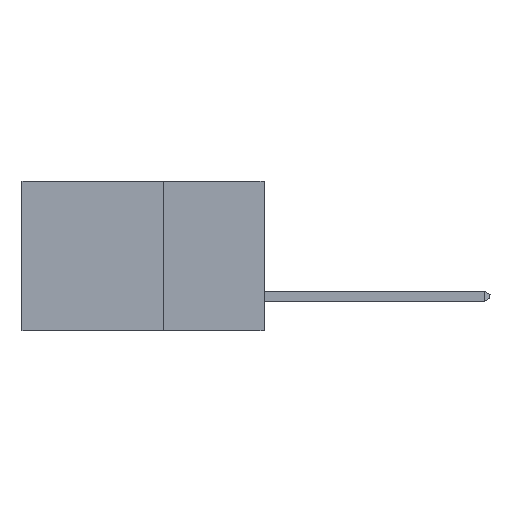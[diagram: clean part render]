
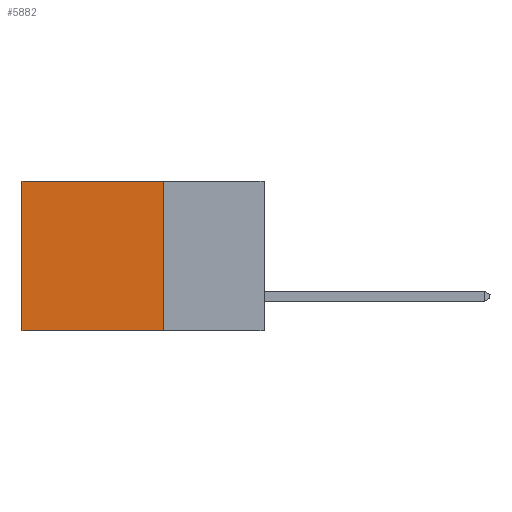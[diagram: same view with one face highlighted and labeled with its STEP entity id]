
A CAD part, left-side view. The second image highlights one B-rep face of the part: STEP entity #5882.
In plain terms, the highlighted planar face has unit normal (-1, 0, 0).
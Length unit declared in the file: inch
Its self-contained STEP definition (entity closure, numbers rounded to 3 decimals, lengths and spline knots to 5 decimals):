
#442 = ORIENTED_EDGE ( 'NONE', *, *, #1939, .T. ) ;
#819 = EDGE_CURVE ( 'NONE', #7518, #7650, #12401, .T. ) ;
#1217 = LINE ( 'NONE', #5498, #1728 ) ;
#1525 = ORIENTED_EDGE ( 'NONE', *, *, #819, .F. ) ;
#1664 = EDGE_LOOP ( 'NONE', ( #442, #1525, #5665, #7998 ) ) ;
#1728 = VECTOR ( 'NONE', #6597, 39.37008 ) ;
#1939 = EDGE_CURVE ( 'NONE', #10340, #7650, #1991, .T. ) ;
#1991 = LINE ( 'NONE', #6845, #7294 ) ;
#2381 = CARTESIAN_POINT ( 'NONE',  ( 0.298, 0.25, 0. ) ) ;
#2501 = DIRECTION ( 'NONE',  ( 0., 0., -1. ) ) ;
#3385 = VECTOR ( 'NONE', #4155, 39.37008 ) ;
#3838 = LINE ( 'NONE', #2381, #13370 ) ;
#4096 = FACE_OUTER_BOUND ( 'NONE', #1664, .T. ) ;
#4155 = DIRECTION ( 'NONE',  ( 0., 1., 0. ) ) ;
#4569 = VERTEX_POINT ( 'NONE', #14044 ) ;
#5196 = EDGE_CURVE ( 'NONE', #4569, #7518, #1217, .T. ) ;
#5498 = CARTESIAN_POINT ( 'NONE',  ( 0.298, 0.25, 0. ) ) ;
#5665 = ORIENTED_EDGE ( 'NONE', *, *, #5196, .F. ) ;
#5820 = PLANE ( 'NONE',  #10823 ) ;
#5882 = ADVANCED_FACE ( 'NONE', ( #4096 ), #5820, .F. ) ;
#6597 = DIRECTION ( 'NONE',  ( 0., 0., -1. ) ) ;
#6845 = CARTESIAN_POINT ( 'NONE',  ( 0.298, 0.6, 0. ) ) ;
#7294 = VECTOR ( 'NONE', #2501, 39.37008 ) ;
#7371 = CARTESIAN_POINT ( 'NONE',  ( 0.298, 0.25, -0.37 ) ) ;
#7518 = VERTEX_POINT ( 'NONE', #9463 ) ;
#7650 = VERTEX_POINT ( 'NONE', #7707 ) ;
#7707 = CARTESIAN_POINT ( 'NONE',  ( 0.298, 0.6, -0.37 ) ) ;
#7998 = ORIENTED_EDGE ( 'NONE', *, *, #14059, .T. ) ;
#9463 = CARTESIAN_POINT ( 'NONE',  ( 0.298, 0.25, -0.37 ) ) ;
#10168 = DIRECTION ( 'NONE',  ( 1., 0., 0. ) ) ;
#10340 = VERTEX_POINT ( 'NONE', #10833 ) ;
#10823 = AXIS2_PLACEMENT_3D ( 'NONE', #11256, #10168, #13459 ) ;
#10833 = CARTESIAN_POINT ( 'NONE',  ( 0.298, 0.6, 0. ) ) ;
#11256 = CARTESIAN_POINT ( 'NONE',  ( 0.298, 0.25, 0. ) ) ;
#12401 = LINE ( 'NONE', #7371, #3385 ) ;
#13215 = DIRECTION ( 'NONE',  ( 0., 1., 0. ) ) ;
#13370 = VECTOR ( 'NONE', #13215, 39.37008 ) ;
#13459 = DIRECTION ( 'NONE',  ( 0., 0., -1. ) ) ;
#14044 = CARTESIAN_POINT ( 'NONE',  ( 0.298, 0.25, 0. ) ) ;
#14059 = EDGE_CURVE ( 'NONE', #4569, #10340, #3838, .T. ) ;
